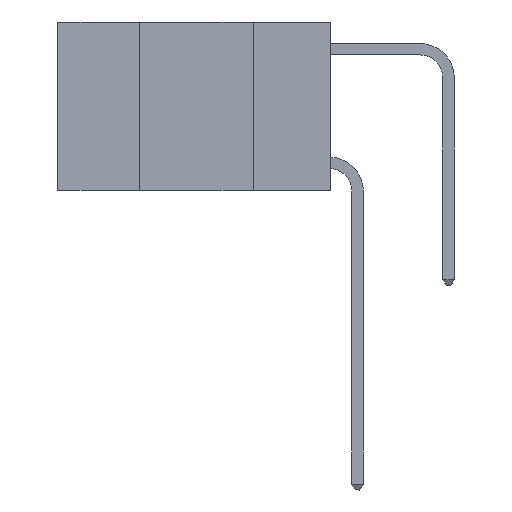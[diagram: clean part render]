
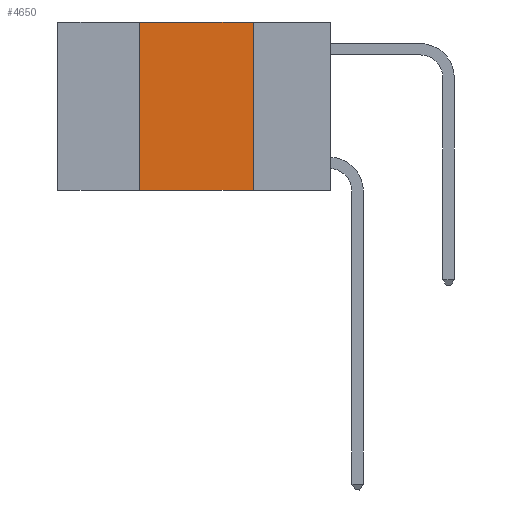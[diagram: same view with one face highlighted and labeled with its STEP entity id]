
A CAD part, left-side view. The second image highlights one B-rep face of the part: STEP entity #4650.
In plain terms, the highlighted planar face has unit normal (-1, 0, 0).
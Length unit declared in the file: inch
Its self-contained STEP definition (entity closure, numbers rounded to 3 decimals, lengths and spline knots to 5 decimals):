
#116 = VECTOR ( 'NONE', #14941, 39.37008 ) ;
#195 = VECTOR ( 'NONE', #2277, 39.37008 ) ;
#1909 = CARTESIAN_POINT ( 'NONE',  ( 0., 0.42, -0.37 ) ) ;
#2277 = DIRECTION ( 'NONE',  ( 0., -1., 0. ) ) ;
#2672 = CARTESIAN_POINT ( 'NONE',  ( 0., 0.17, 0. ) ) ;
#2737 = ORIENTED_EDGE ( 'NONE', *, *, #17270, .F. ) ;
#2901 = ORIENTED_EDGE ( 'NONE', *, *, #14155, .F. ) ;
#2937 = ORIENTED_EDGE ( 'NONE', *, *, #6486, .F. ) ;
#2939 = CARTESIAN_POINT ( 'NONE',  ( 0., 0.42, 0. ) ) ;
#3098 = ORIENTED_EDGE ( 'NONE', *, *, #13063, .T. ) ;
#3137 = VERTEX_POINT ( 'NONE', #1909 ) ;
#3185 = FACE_OUTER_BOUND ( 'NONE', #17277, .T. ) ;
#4178 = LINE ( 'NONE', #11963, #116 ) ;
#4650 = ADVANCED_FACE ( 'NONE', ( #3185 ), #15001, .F. ) ;
#5398 = CARTESIAN_POINT ( 'NONE',  ( 0., 0.6, -0.37 ) ) ;
#6293 = CARTESIAN_POINT ( 'NONE',  ( 0., 0.6, 0. ) ) ;
#6486 = EDGE_CURVE ( 'NONE', #3137, #9433, #17706, .T. ) ;
#7146 = LINE ( 'NONE', #14004, #17279 ) ;
#7800 = DIRECTION ( 'NONE',  ( 0., 0., -1. ) ) ;
#9433 = VERTEX_POINT ( 'NONE', #17347 ) ;
#9501 = VERTEX_POINT ( 'NONE', #10264 ) ;
#10264 = CARTESIAN_POINT ( 'NONE',  ( 0., 0.17, -0.37 ) ) ;
#11580 = LINE ( 'NONE', #5398, #195 ) ;
#11963 = CARTESIAN_POINT ( 'NONE',  ( 0., 0.6, 0. ) ) ;
#13063 = EDGE_CURVE ( 'NONE', #3137, #9501, #11580, .T. ) ;
#13876 = VECTOR ( 'NONE', #17544, 39.37008 ) ;
#14004 = CARTESIAN_POINT ( 'NONE',  ( 0., 0.17, 0. ) ) ;
#14155 = EDGE_CURVE ( 'NONE', #9433, #14625, #4178, .T. ) ;
#14625 = VERTEX_POINT ( 'NONE', #2672 ) ;
#14941 = DIRECTION ( 'NONE',  ( 0., -1., 0. ) ) ;
#15001 = PLANE ( 'NONE',  #15766 ) ;
#15766 = AXIS2_PLACEMENT_3D ( 'NONE', #6293, #16434, #7800 ) ;
#16434 = DIRECTION ( 'NONE',  ( 1., 0., 0. ) ) ;
#16837 = DIRECTION ( 'NONE',  ( 0., 0., -1. ) ) ;
#17270 = EDGE_CURVE ( 'NONE', #14625, #9501, #7146, .T. ) ;
#17277 = EDGE_LOOP ( 'NONE', ( #2737, #2901, #2937, #3098 ) ) ;
#17279 = VECTOR ( 'NONE', #16837, 39.37008 ) ;
#17347 = CARTESIAN_POINT ( 'NONE',  ( 0., 0.42, 0. ) ) ;
#17544 = DIRECTION ( 'NONE',  ( 0., 0., 1. ) ) ;
#17706 = LINE ( 'NONE', #2939, #13876 ) ;
